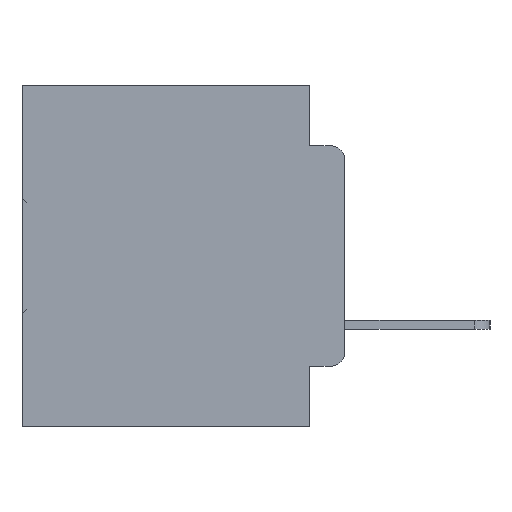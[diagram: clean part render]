
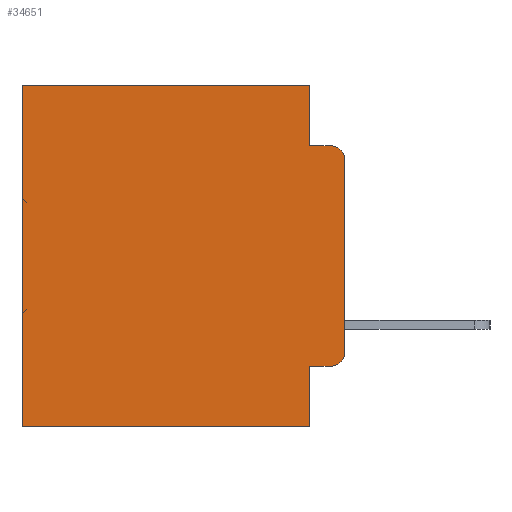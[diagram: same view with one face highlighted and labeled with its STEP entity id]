
A CAD part, left-side view. The second image highlights one B-rep face of the part: STEP entity #34651.
In plain terms, the highlighted planar face has unit normal (-1, 0, 0).
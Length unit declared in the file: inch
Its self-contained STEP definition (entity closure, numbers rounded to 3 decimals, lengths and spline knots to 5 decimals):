
#927 = VERTEX_POINT ( 'NONE', #11865 ) ;
#936 = CARTESIAN_POINT ( 'NONE',  ( 0.298, 0., -0.5 ) ) ;
#1130 = EDGE_LOOP ( 'NONE', ( #14062, #17960, #23397, #3439, #3732, #5044, #12259, #17322, #31337, #16049 ) ) ;
#1378 = CIRCLE ( 'NONE', #28946, 0.02 ) ;
#1893 = DIRECTION ( 'NONE',  ( 0., 0., -1. ) ) ;
#2378 = VERTEX_POINT ( 'NONE', #7605 ) ;
#2646 = EDGE_CURVE ( 'NONE', #927, #7237, #21151, .T. ) ;
#3322 = VERTEX_POINT ( 'NONE', #28424 ) ;
#3439 = ORIENTED_EDGE ( 'NONE', *, *, #11857, .F. ) ;
#3450 = EDGE_CURVE ( 'NONE', #3322, #7237, #26116, .T. ) ;
#3722 = DIRECTION ( 'NONE',  ( 0., 0., -1. ) ) ;
#3732 = ORIENTED_EDGE ( 'NONE', *, *, #6329, .T. ) ;
#4724 = EDGE_CURVE ( 'NONE', #11143, #3322, #13380, .T. ) ;
#5044 = ORIENTED_EDGE ( 'NONE', *, *, #2646, .T. ) ;
#5058 = DIRECTION ( 'NONE',  ( -1., 0., 0. ) ) ;
#5969 = CARTESIAN_POINT ( 'NONE',  ( 0.298, 0.02, -0.3915 ) ) ;
#6043 = AXIS2_PLACEMENT_3D ( 'NONE', #21350, #5058, #24089 ) ;
#6291 = DIRECTION ( 'NONE',  ( 0., 1., 0. ) ) ;
#6329 = EDGE_CURVE ( 'NONE', #33850, #927, #8567, .T. ) ;
#6831 = VECTOR ( 'NONE', #19702, 39.37008 ) ;
#6846 = EDGE_CURVE ( 'NONE', #2378, #8998, #14058, .T. ) ;
#7185 = LINE ( 'NONE', #29235, #34686 ) ;
#7237 = VERTEX_POINT ( 'NONE', #10399 ) ;
#7605 = CARTESIAN_POINT ( 'NONE',  ( 0.298, 0.051, -0.0885 ) ) ;
#7876 = CARTESIAN_POINT ( 'NONE',  ( 0.298, 0.02, -0.4115 ) ) ;
#7926 = VERTEX_POINT ( 'NONE', #18822 ) ;
#8150 = CARTESIAN_POINT ( 'NONE',  ( 0.298, 0.473, 0. ) ) ;
#8390 = CARTESIAN_POINT ( 'NONE',  ( 0.298, 0.051, 0. ) ) ;
#8567 = LINE ( 'NONE', #22568, #29965 ) ;
#8712 = DIRECTION ( 'NONE',  ( 0., 0., -1. ) ) ;
#8998 = VERTEX_POINT ( 'NONE', #29035 ) ;
#9096 = DIRECTION ( 'NONE',  ( 0., 0., -1. ) ) ;
#10399 = CARTESIAN_POINT ( 'NONE',  ( 0.298, 0.473, -0.5 ) ) ;
#10949 = EDGE_CURVE ( 'NONE', #22671, #7926, #7185, .T. ) ;
#11143 = VERTEX_POINT ( 'NONE', #19483 ) ;
#11857 = EDGE_CURVE ( 'NONE', #33850, #2378, #13982, .T. ) ;
#11865 = CARTESIAN_POINT ( 'NONE',  ( 0.298, 0.473, 0. ) ) ;
#12259 = ORIENTED_EDGE ( 'NONE', *, *, #3450, .F. ) ;
#12326 = EDGE_CURVE ( 'NONE', #22671, #8998, #13114, .T. ) ;
#12534 = VECTOR ( 'NONE', #3722, 39.37008 ) ;
#12935 = CARTESIAN_POINT ( 'NONE',  ( 0.298, 0.051, -0.4115 ) ) ;
#13114 = CIRCLE ( 'NONE', #6043, 0.02 ) ;
#13380 = LINE ( 'NONE', #19891, #12534 ) ;
#13982 = LINE ( 'NONE', #19284, #20344 ) ;
#14058 = LINE ( 'NONE', #22302, #6831 ) ;
#14062 = ORIENTED_EDGE ( 'NONE', *, *, #10949, .F. ) ;
#15659 = VECTOR ( 'NONE', #9096, 39.37008 ) ;
#16049 = ORIENTED_EDGE ( 'NONE', *, *, #24307, .T. ) ;
#17322 = ORIENTED_EDGE ( 'NONE', *, *, #4724, .F. ) ;
#17960 = ORIENTED_EDGE ( 'NONE', *, *, #12326, .T. ) ;
#18304 = DIRECTION ( 'NONE',  ( 1., 0., 0. ) ) ;
#18822 = CARTESIAN_POINT ( 'NONE',  ( 0.298, 0., -0.3915 ) ) ;
#19284 = CARTESIAN_POINT ( 'NONE',  ( 0.298, 0.051, 0. ) ) ;
#19483 = CARTESIAN_POINT ( 'NONE',  ( 0.298, 0.051, -0.4115 ) ) ;
#19702 = DIRECTION ( 'NONE',  ( 0., -1., 0. ) ) ;
#19891 = CARTESIAN_POINT ( 'NONE',  ( 0.298, 0.051, 0. ) ) ;
#19980 = VERTEX_POINT ( 'NONE', #7876 ) ;
#20344 = VECTOR ( 'NONE', #27297, 39.37008 ) ;
#21151 = LINE ( 'NONE', #8150, #15659 ) ;
#21350 = CARTESIAN_POINT ( 'NONE',  ( 0.298, 0.02, -0.1085 ) ) ;
#22302 = CARTESIAN_POINT ( 'NONE',  ( 0.298, 0.051, -0.0885 ) ) ;
#22568 = CARTESIAN_POINT ( 'NONE',  ( 0.298, 0., 0. ) ) ;
#22671 = VERTEX_POINT ( 'NONE', #34579 ) ;
#23397 = ORIENTED_EDGE ( 'NONE', *, *, #6846, .F. ) ;
#24089 = DIRECTION ( 'NONE',  ( 0., 0., -1. ) ) ;
#24307 = EDGE_CURVE ( 'NONE', #19980, #7926, #1378, .T. ) ;
#24943 = DIRECTION ( 'NONE',  ( -1., 0., 0. ) ) ;
#26116 = LINE ( 'NONE', #936, #30583 ) ;
#26739 = FACE_OUTER_BOUND ( 'NONE', #1130, .T. ) ;
#27297 = DIRECTION ( 'NONE',  ( 0., 0., -1. ) ) ;
#28074 = AXIS2_PLACEMENT_3D ( 'NONE', #28878, #18304, #1893 ) ;
#28424 = CARTESIAN_POINT ( 'NONE',  ( 0.298, 0.051, -0.5 ) ) ;
#28764 = PLANE ( 'NONE',  #28074 ) ;
#28878 = CARTESIAN_POINT ( 'NONE',  ( 0.298, 0., 0. ) ) ;
#28946 = AXIS2_PLACEMENT_3D ( 'NONE', #5969, #24943, #8712 ) ;
#28992 = DIRECTION ( 'NONE',  ( 0., -1., 0. ) ) ;
#29035 = CARTESIAN_POINT ( 'NONE',  ( 0.298, 0.02, -0.0885 ) ) ;
#29235 = CARTESIAN_POINT ( 'NONE',  ( 0.298, 0., 0. ) ) ;
#29965 = VECTOR ( 'NONE', #6291, 39.37008 ) ;
#30583 = VECTOR ( 'NONE', #33245, 39.37008 ) ;
#31337 = ORIENTED_EDGE ( 'NONE', *, *, #34680, .T. ) ;
#31812 = DIRECTION ( 'NONE',  ( 0., 0., -1. ) ) ;
#32784 = LINE ( 'NONE', #12935, #33595 ) ;
#33245 = DIRECTION ( 'NONE',  ( 0., 1., 0. ) ) ;
#33595 = VECTOR ( 'NONE', #28992, 39.37008 ) ;
#33850 = VERTEX_POINT ( 'NONE', #8390 ) ;
#34579 = CARTESIAN_POINT ( 'NONE',  ( 0.298, 0., -0.1085 ) ) ;
#34651 = ADVANCED_FACE ( 'NONE', ( #26739 ), #28764, .F. ) ;
#34680 = EDGE_CURVE ( 'NONE', #11143, #19980, #32784, .T. ) ;
#34686 = VECTOR ( 'NONE', #31812, 39.37008 ) ;
